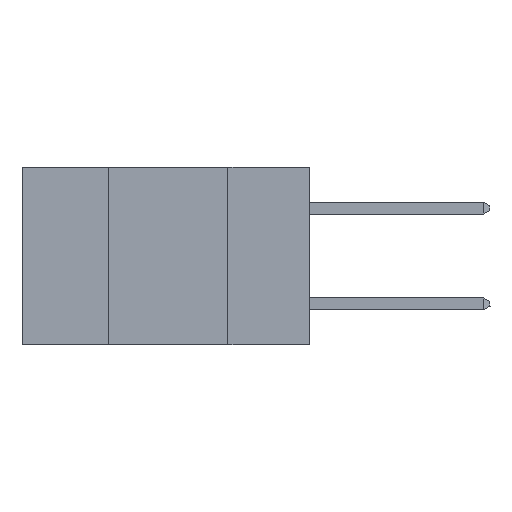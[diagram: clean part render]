
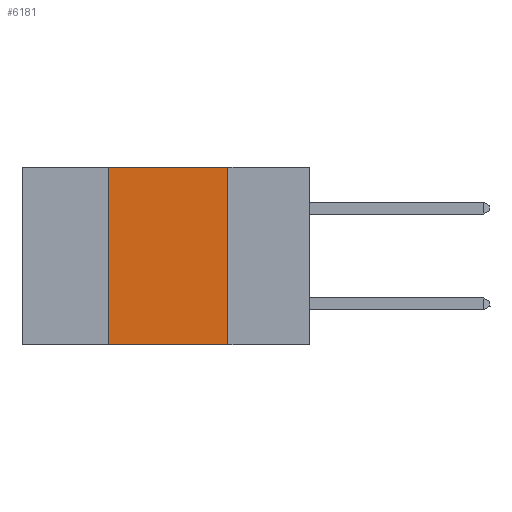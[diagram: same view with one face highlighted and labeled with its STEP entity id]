
A CAD part, left-side view. The second image highlights one B-rep face of the part: STEP entity #6181.
In plain terms, the highlighted planar face has unit normal (-1, 0, 0).
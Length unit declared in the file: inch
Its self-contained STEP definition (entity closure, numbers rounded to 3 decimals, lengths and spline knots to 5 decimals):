
#672 = EDGE_LOOP ( 'NONE', ( #8268, #9981, #7762, #11946 ) ) ;
#909 = EDGE_CURVE ( 'NONE', #15239, #6754, #1512, .T. ) ;
#1512 = LINE ( 'NONE', #4217, #11808 ) ;
#1766 = DIRECTION ( 'NONE',  ( 0., 0., 1. ) ) ;
#2302 = VERTEX_POINT ( 'NONE', #8235 ) ;
#2731 = LINE ( 'NONE', #12267, #9126 ) ;
#2738 = DIRECTION ( 'NONE',  ( 0., 0., -1. ) ) ;
#3146 = DIRECTION ( 'NONE',  ( 0., -1., 0. ) ) ;
#3330 = VECTOR ( 'NONE', #14577, 39.37008 ) ;
#3881 = VERTEX_POINT ( 'NONE', #7484 ) ;
#3949 = VECTOR ( 'NONE', #3146, 39.37008 ) ;
#3984 = CARTESIAN_POINT ( 'NONE',  ( 0., 0.42, -0.37 ) ) ;
#4217 = CARTESIAN_POINT ( 'NONE',  ( 0., 0.42, 0. ) ) ;
#4480 = DIRECTION ( 'NONE',  ( 1., 0., 0. ) ) ;
#5867 = EDGE_CURVE ( 'NONE', #6754, #3881, #9721, .T. ) ;
#6181 = ADVANCED_FACE ( 'NONE', ( #8379 ), #11614, .F. ) ;
#6249 = CARTESIAN_POINT ( 'NONE',  ( 0., 0.6, 0. ) ) ;
#6575 = EDGE_CURVE ( 'NONE', #3881, #2302, #2731, .T. ) ;
#6697 = CARTESIAN_POINT ( 'NONE',  ( 0., 0.6, -0.37 ) ) ;
#6754 = VERTEX_POINT ( 'NONE', #10288 ) ;
#7484 = CARTESIAN_POINT ( 'NONE',  ( 0., 0.17, 0. ) ) ;
#7762 = ORIENTED_EDGE ( 'NONE', *, *, #909, .F. ) ;
#8038 = CARTESIAN_POINT ( 'NONE',  ( 0., 0.6, 0. ) ) ;
#8235 = CARTESIAN_POINT ( 'NONE',  ( 0., 0.17, -0.37 ) ) ;
#8268 = ORIENTED_EDGE ( 'NONE', *, *, #6575, .F. ) ;
#8379 = FACE_OUTER_BOUND ( 'NONE', #672, .T. ) ;
#9126 = VECTOR ( 'NONE', #2738, 39.37008 ) ;
#9133 = AXIS2_PLACEMENT_3D ( 'NONE', #8038, #4480, #12794 ) ;
#9721 = LINE ( 'NONE', #6249, #3330 ) ;
#9981 = ORIENTED_EDGE ( 'NONE', *, *, #5867, .F. ) ;
#10288 = CARTESIAN_POINT ( 'NONE',  ( 0., 0.42, 0. ) ) ;
#11614 = PLANE ( 'NONE',  #9133 ) ;
#11808 = VECTOR ( 'NONE', #1766, 39.37008 ) ;
#11946 = ORIENTED_EDGE ( 'NONE', *, *, #15419, .T. ) ;
#12267 = CARTESIAN_POINT ( 'NONE',  ( 0., 0.17, 0. ) ) ;
#12794 = DIRECTION ( 'NONE',  ( 0., 0., -1. ) ) ;
#13419 = LINE ( 'NONE', #6697, #3949 ) ;
#14577 = DIRECTION ( 'NONE',  ( 0., -1., 0. ) ) ;
#15239 = VERTEX_POINT ( 'NONE', #3984 ) ;
#15419 = EDGE_CURVE ( 'NONE', #15239, #2302, #13419, .T. ) ;
